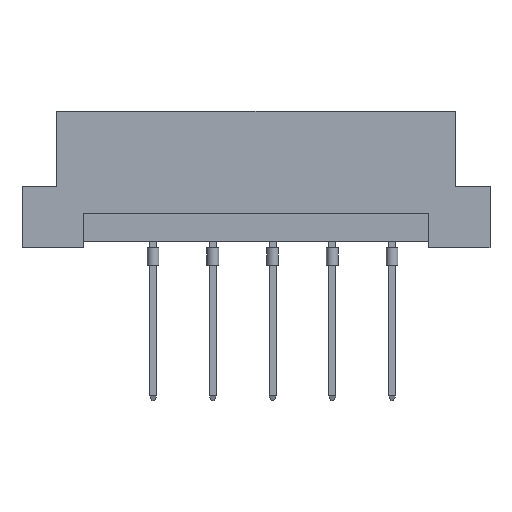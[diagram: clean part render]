
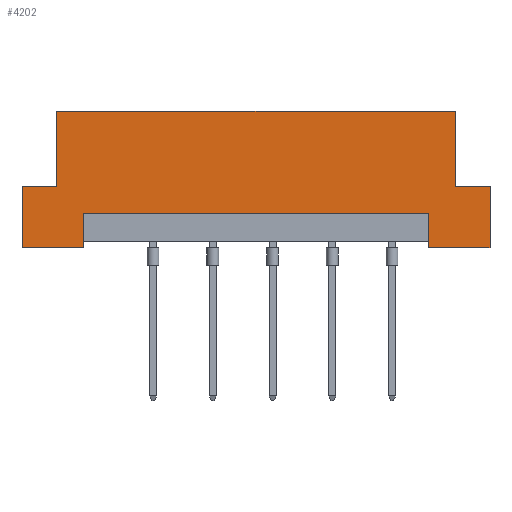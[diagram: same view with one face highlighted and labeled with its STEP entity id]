
A CAD part, front view. The second image highlights one B-rep face of the part: STEP entity #4202.
In plain terms, the highlighted planar face has unit normal (0, -1, 0).
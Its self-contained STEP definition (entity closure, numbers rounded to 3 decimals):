
#11 = VECTOR ( 'NONE', #4161, 1000. ) ;
#49 = LINE ( 'NONE', #155, #6747 ) ;
#81 = CARTESIAN_POINT ( 'NONE',  ( 14.69, 0., 0.5 ) ) ;
#155 = CARTESIAN_POINT ( 'NONE',  ( 16.94, 0., 5.2 ) ) ;
#196 = CARTESIAN_POINT ( 'NONE',  ( 19.9, 0., 5.2 ) ) ;
#223 = LINE ( 'NONE', #3470, #4547 ) ;
#226 = ORIENTED_EDGE ( 'NONE', *, *, #291, .F. ) ;
#267 = VERTEX_POINT ( 'NONE', #5806 ) ;
#291 = EDGE_CURVE ( 'NONE', #5495, #5055, #2682, .T. ) ;
#475 = CARTESIAN_POINT ( 'NONE',  ( -19.9, 0., 5.2 ) ) ;
#580 = AXIS2_PLACEMENT_3D ( 'NONE', #4369, #5988, #4971 ) ;
#598 = LINE ( 'NONE', #3299, #4792 ) ;
#626 = VERTEX_POINT ( 'NONE', #196 ) ;
#755 = DIRECTION ( 'NONE',  ( 0., 0., -1. ) ) ;
#773 = EDGE_CURVE ( 'NONE', #4753, #3265, #3215, .T. ) ;
#784 = EDGE_CURVE ( 'NONE', #626, #7048, #1981, .T. ) ;
#973 = DIRECTION ( 'NONE',  ( -1., 0., 0. ) ) ;
#1077 = DIRECTION ( 'NONE',  ( 0., 0., -1. ) ) ;
#1083 = VERTEX_POINT ( 'NONE', #1894 ) ;
#1109 = LINE ( 'NONE', #81, #2184 ) ;
#1275 = ORIENTED_EDGE ( 'NONE', *, *, #773, .F. ) ;
#1440 = DIRECTION ( 'NONE',  ( 0., 0., -1. ) ) ;
#1514 = EDGE_CURVE ( 'NONE', #4699, #626, #3087, .T. ) ;
#1532 = CARTESIAN_POINT ( 'NONE',  ( 14.69, 0., 0. ) ) ;
#1682 = ORIENTED_EDGE ( 'NONE', *, *, #3506, .T. ) ;
#1706 = ORIENTED_EDGE ( 'NONE', *, *, #5999, .F. ) ;
#1766 = DIRECTION ( 'NONE',  ( 1., 0., 0. ) ) ;
#1894 = CARTESIAN_POINT ( 'NONE',  ( -19.9, 0., 0. ) ) ;
#1981 = LINE ( 'NONE', #6343, #5599 ) ;
#2047 = CARTESIAN_POINT ( 'NONE',  ( -19.9, 0., 0. ) ) ;
#2074 = VERTEX_POINT ( 'NONE', #475 ) ;
#2184 = VECTOR ( 'NONE', #1077, 1000. ) ;
#2197 = FACE_OUTER_BOUND ( 'NONE', #3164, .T. ) ;
#2368 = ORIENTED_EDGE ( 'NONE', *, *, #3722, .F. ) ;
#2443 = DIRECTION ( 'NONE',  ( 1., 0., 0. ) ) ;
#2682 = LINE ( 'NONE', #3187, #4705 ) ;
#2799 = ORIENTED_EDGE ( 'NONE', *, *, #6370, .T. ) ;
#2882 = CARTESIAN_POINT ( 'NONE',  ( -16.94, 0., 11.6 ) ) ;
#3019 = CARTESIAN_POINT ( 'NONE',  ( 19.9, 0., 0. ) ) ;
#3056 = EDGE_CURVE ( 'NONE', #2074, #5495, #5439, .T. ) ;
#3078 = CARTESIAN_POINT ( 'NONE',  ( -14.69, 0., 2.9 ) ) ;
#3087 = LINE ( 'NONE', #5264, #5314 ) ;
#3114 = LINE ( 'NONE', #2047, #11 ) ;
#3164 = EDGE_LOOP ( 'NONE', ( #1275, #2799, #3230, #3491, #5215, #1682, #1706, #226, #5522, #6054, #5443, #2368 ) ) ;
#3187 = CARTESIAN_POINT ( 'NONE',  ( -16.94, 0., 5.2 ) ) ;
#3196 = CARTESIAN_POINT ( 'NONE',  ( -16.94, 0., 5.2 ) ) ;
#3215 = LINE ( 'NONE', #4154, #6404 ) ;
#3230 = ORIENTED_EDGE ( 'NONE', *, *, #4556, .F. ) ;
#3265 = VERTEX_POINT ( 'NONE', #3078 ) ;
#3299 = CARTESIAN_POINT ( 'NONE',  ( -19.9, 0., 0. ) ) ;
#3470 = CARTESIAN_POINT ( 'NONE',  ( -14.69, 0., 0.5 ) ) ;
#3491 = ORIENTED_EDGE ( 'NONE', *, *, #784, .F. ) ;
#3506 = EDGE_CURVE ( 'NONE', #4699, #5653, #49, .T. ) ;
#3722 = EDGE_CURVE ( 'NONE', #3265, #267, #223, .T. ) ;
#3774 = VECTOR ( 'NONE', #6932, 1000. ) ;
#3832 = CARTESIAN_POINT ( 'NONE',  ( -19.9, 0., 11.6 ) ) ;
#3911 = DIRECTION ( 'NONE',  ( 0., 0., 1. ) ) ;
#3933 = DIRECTION ( 'NONE',  ( 0., 0., 1. ) ) ;
#4154 = CARTESIAN_POINT ( 'NONE',  ( 14.69, 0., 2.9 ) ) ;
#4161 = DIRECTION ( 'NONE',  ( -1., 0., 0. ) ) ;
#4202 = ADVANCED_FACE ( 'NONE', ( #2197 ), #4899, .F. ) ;
#4323 = CARTESIAN_POINT ( 'NONE',  ( 16.94, 0., 5.2 ) ) ;
#4369 = CARTESIAN_POINT ( 'NONE',  ( -19.9, 0., 11.6 ) ) ;
#4439 = EDGE_CURVE ( 'NONE', #267, #1083, #3114, .T. ) ;
#4464 = DIRECTION ( 'NONE',  ( 1., 0., 0. ) ) ;
#4547 = VECTOR ( 'NONE', #755, 1000. ) ;
#4556 = EDGE_CURVE ( 'NONE', #7048, #4962, #4784, .T. ) ;
#4561 = CARTESIAN_POINT ( 'NONE',  ( 14.69, 0., 2.9 ) ) ;
#4620 = CARTESIAN_POINT ( 'NONE',  ( 16.94, 0., 11.6 ) ) ;
#4699 = VERTEX_POINT ( 'NONE', #4323 ) ;
#4705 = VECTOR ( 'NONE', #5370, 1000. ) ;
#4722 = CARTESIAN_POINT ( 'NONE',  ( -19.9, 0., 0. ) ) ;
#4753 = VERTEX_POINT ( 'NONE', #4561 ) ;
#4784 = LINE ( 'NONE', #4722, #3774 ) ;
#4792 = VECTOR ( 'NONE', #3911, 1000. ) ;
#4888 = LINE ( 'NONE', #3832, #6179 ) ;
#4899 = PLANE ( 'NONE',  #580 ) ;
#4962 = VERTEX_POINT ( 'NONE', #1532 ) ;
#4971 = DIRECTION ( 'NONE',  ( 0., 0., 1. ) ) ;
#5055 = VERTEX_POINT ( 'NONE', #2882 ) ;
#5215 = ORIENTED_EDGE ( 'NONE', *, *, #1514, .F. ) ;
#5264 = CARTESIAN_POINT ( 'NONE',  ( 19.9, 0., 5.2 ) ) ;
#5314 = VECTOR ( 'NONE', #2443, 1000. ) ;
#5370 = DIRECTION ( 'NONE',  ( 0., 0., 1. ) ) ;
#5439 = LINE ( 'NONE', #6053, #5812 ) ;
#5443 = ORIENTED_EDGE ( 'NONE', *, *, #4439, .F. ) ;
#5495 = VERTEX_POINT ( 'NONE', #3196 ) ;
#5522 = ORIENTED_EDGE ( 'NONE', *, *, #3056, .F. ) ;
#5546 = EDGE_CURVE ( 'NONE', #1083, #2074, #598, .T. ) ;
#5599 = VECTOR ( 'NONE', #1440, 1000. ) ;
#5653 = VERTEX_POINT ( 'NONE', #4620 ) ;
#5806 = CARTESIAN_POINT ( 'NONE',  ( -14.69, 0., 0. ) ) ;
#5812 = VECTOR ( 'NONE', #1766, 1000. ) ;
#5988 = DIRECTION ( 'NONE',  ( 0., 1., 0. ) ) ;
#5999 = EDGE_CURVE ( 'NONE', #5055, #5653, #4888, .T. ) ;
#6053 = CARTESIAN_POINT ( 'NONE',  ( -19.9, 0., 5.2 ) ) ;
#6054 = ORIENTED_EDGE ( 'NONE', *, *, #5546, .F. ) ;
#6179 = VECTOR ( 'NONE', #4464, 1000. ) ;
#6343 = CARTESIAN_POINT ( 'NONE',  ( 19.9, 0., 0. ) ) ;
#6370 = EDGE_CURVE ( 'NONE', #4753, #4962, #1109, .T. ) ;
#6404 = VECTOR ( 'NONE', #973, 1000. ) ;
#6747 = VECTOR ( 'NONE', #3933, 1000. ) ;
#6932 = DIRECTION ( 'NONE',  ( -1., 0., 0. ) ) ;
#7048 = VERTEX_POINT ( 'NONE', #3019 ) ;
